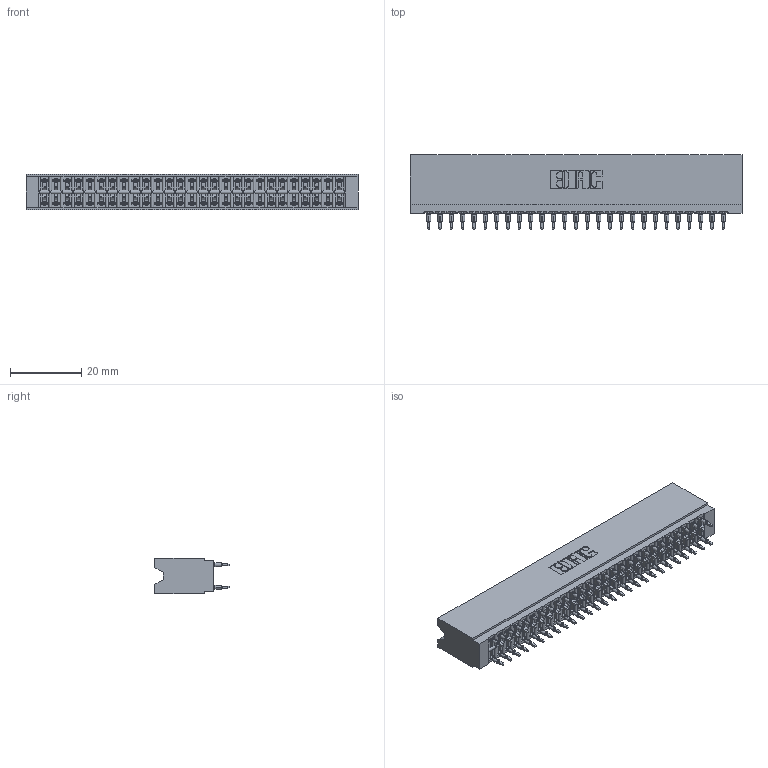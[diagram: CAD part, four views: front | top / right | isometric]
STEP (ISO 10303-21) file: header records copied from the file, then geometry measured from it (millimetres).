
FILE_DESCRIPTION (( 'STEP AP203' ), '1' );
FILE_NAME ('746-054-560-206.STEP', '2026-02-27T19:35:47', ( '' ), ( '' ), 'SwSTEP 2.0', 'SolidWorks 2023', '' );
FILE_SCHEMA (( 'CONFIG_CONTROL_DESIGN' ));
Length unit declared in the file: millimetre
Products named in the file (3): 746-292-001_560; 746-054-560-206; 746 Part_.515 Slot Depth - 06
Assembly tree (55 placements, depth 2):
  746-054-560-206
    746 Part_.515 Slot Depth - 06
    746-292-001_560  x54
Bounding box: 92.96 x 20.82 x 9.91 mm (x, y, z)
Volume: 10225.4 mm3; surface area: 17017.3 mm2
Topology: 55 solids, 55 shells, 5201 faces, 14467 edges, 9274 vertices
Faces by surface type: plane 2594, cylinder 1203, bspline 1080, torus 324
Entity records: 43990 total; most frequent: CARTESIAN_POINT 8872, ORIENTED_EDGE 7522, DIRECTION 6313, EDGE_CURVE 3761, LINE 3299, VECTOR 3299, VERTEX_POINT 2490, AXIS2_PLACEMENT_3D 1507
